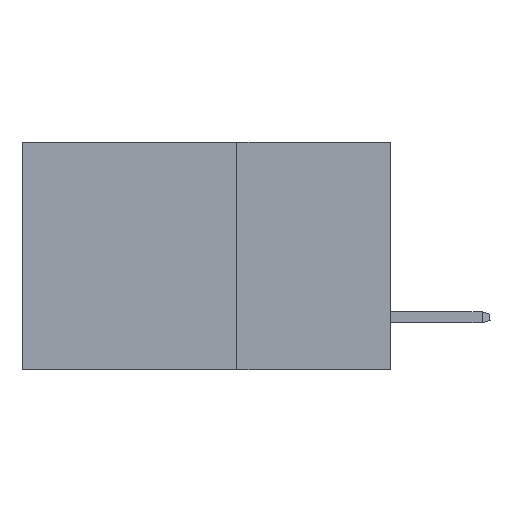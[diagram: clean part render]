
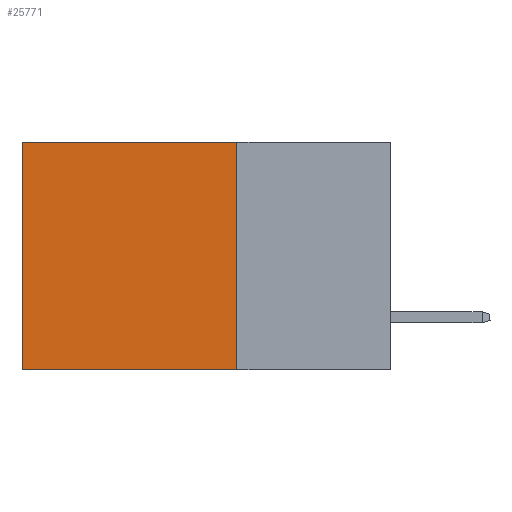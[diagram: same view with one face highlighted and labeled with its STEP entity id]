
A CAD part, left-side view. The second image highlights one B-rep face of the part: STEP entity #25771.
In plain terms, the highlighted planar face has unit normal (-1, 0, 0).
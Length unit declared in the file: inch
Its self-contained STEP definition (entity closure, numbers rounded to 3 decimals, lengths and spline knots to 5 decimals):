
#666 = CARTESIAN_POINT ( 'NONE',  ( 0.2875, 0.25, -0.37 ) ) ;
#3856 = VERTEX_POINT ( 'NONE', #13403 ) ;
#3876 = DIRECTION ( 'NONE',  ( 0., 1., 0. ) ) ;
#4276 = VERTEX_POINT ( 'NONE', #19611 ) ;
#6674 = ORIENTED_EDGE ( 'NONE', *, *, #21949, .F. ) ;
#8315 = EDGE_CURVE ( 'NONE', #3856, #12290, #15168, .T. ) ;
#8379 = VECTOR ( 'NONE', #40747, 39.37008 ) ;
#9933 = EDGE_CURVE ( 'NONE', #10145, #4276, #20940, .T. ) ;
#10145 = VERTEX_POINT ( 'NONE', #22226 ) ;
#10915 = CARTESIAN_POINT ( 'NONE',  ( 0.2875, 0.6, -0.37 ) ) ;
#10965 = DIRECTION ( 'NONE',  ( 0., 0., -1. ) ) ;
#12290 = VERTEX_POINT ( 'NONE', #10915 ) ;
#13017 = PLANE ( 'NONE',  #13635 ) ;
#13403 = CARTESIAN_POINT ( 'NONE',  ( 0.2875, 0.6, 0. ) ) ;
#13635 = AXIS2_PLACEMENT_3D ( 'NONE', #38721, #29342, #19494 ) ;
#15168 = LINE ( 'NONE', #26970, #41271 ) ;
#15818 = LINE ( 'NONE', #23748, #20862 ) ;
#17271 = EDGE_LOOP ( 'NONE', ( #29471, #6674, #38069, #21547 ) ) ;
#17775 = FACE_OUTER_BOUND ( 'NONE', #17271, .T. ) ;
#19494 = DIRECTION ( 'NONE',  ( 0., 0., -1. ) ) ;
#19611 = CARTESIAN_POINT ( 'NONE',  ( 0.2875, 0.25, -0.37 ) ) ;
#20862 = VECTOR ( 'NONE', #33458, 39.37008 ) ;
#20940 = LINE ( 'NONE', #40092, #8379 ) ;
#21547 = ORIENTED_EDGE ( 'NONE', *, *, #39324, .T. ) ;
#21949 = EDGE_CURVE ( 'NONE', #4276, #12290, #38594, .T. ) ;
#22226 = CARTESIAN_POINT ( 'NONE',  ( 0.2875, 0.25, 0. ) ) ;
#23748 = CARTESIAN_POINT ( 'NONE',  ( 0.2875, 0.25, 0. ) ) ;
#25771 = ADVANCED_FACE ( 'NONE', ( #17775 ), #13017, .F. ) ;
#26970 = CARTESIAN_POINT ( 'NONE',  ( 0.2875, 0.6, 0. ) ) ;
#29342 = DIRECTION ( 'NONE',  ( 1., 0., 0. ) ) ;
#29471 = ORIENTED_EDGE ( 'NONE', *, *, #8315, .T. ) ;
#33103 = VECTOR ( 'NONE', #3876, 39.37008 ) ;
#33458 = DIRECTION ( 'NONE',  ( 0., 1., 0. ) ) ;
#38069 = ORIENTED_EDGE ( 'NONE', *, *, #9933, .F. ) ;
#38594 = LINE ( 'NONE', #666, #33103 ) ;
#38721 = CARTESIAN_POINT ( 'NONE',  ( 0.2875, 0.25, 0. ) ) ;
#39324 = EDGE_CURVE ( 'NONE', #10145, #3856, #15818, .T. ) ;
#40092 = CARTESIAN_POINT ( 'NONE',  ( 0.2875, 0.25, 0. ) ) ;
#40747 = DIRECTION ( 'NONE',  ( 0., 0., -1. ) ) ;
#41271 = VECTOR ( 'NONE', #10965, 39.37008 ) ;
